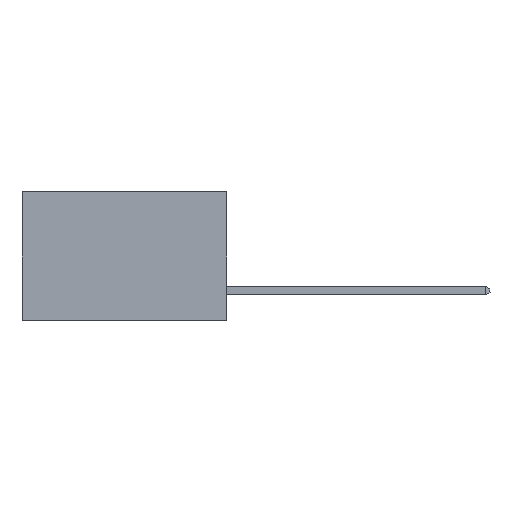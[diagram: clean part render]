
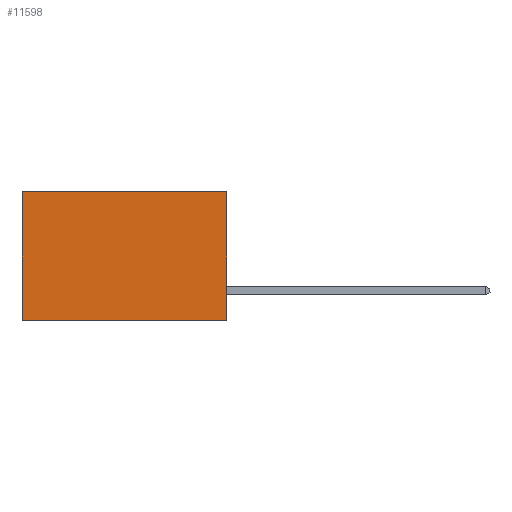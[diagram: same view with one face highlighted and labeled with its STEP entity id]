
A CAD part, left-side view. The second image highlights one B-rep face of the part: STEP entity #11598.
In plain terms, the highlighted planar face has unit normal (-1, 0, 0).
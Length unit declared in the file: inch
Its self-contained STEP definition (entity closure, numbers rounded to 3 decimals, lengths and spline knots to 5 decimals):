
#494 = VERTEX_POINT ( 'NONE', #1465 ) ;
#564 = EDGE_LOOP ( 'NONE', ( #7076, #9869, #7404, #1707 ) ) ;
#666 = EDGE_CURVE ( 'NONE', #3125, #494, #12591, .T. ) ;
#913 = CARTESIAN_POINT ( 'NONE',  ( 0.277, 0., -0.37 ) ) ;
#1465 = CARTESIAN_POINT ( 'NONE',  ( 0.277, 0.59, -0.37 ) ) ;
#1583 = DIRECTION ( 'NONE',  ( 0., 1., 0. ) ) ;
#1707 = ORIENTED_EDGE ( 'NONE', *, *, #13113, .T. ) ;
#2767 = CARTESIAN_POINT ( 'NONE',  ( 0.277, 0., 0. ) ) ;
#3125 = VERTEX_POINT ( 'NONE', #10188 ) ;
#3278 = DIRECTION ( 'NONE',  ( 0., 0., -1. ) ) ;
#3287 = VECTOR ( 'NONE', #5679, 39.37008 ) ;
#3645 = AXIS2_PLACEMENT_3D ( 'NONE', #913, #9851, #3278 ) ;
#3922 = VECTOR ( 'NONE', #1583, 39.37008 ) ;
#4216 = DIRECTION ( 'NONE',  ( 0., 0., -1. ) ) ;
#4463 = DIRECTION ( 'NONE',  ( 0., 1., 0. ) ) ;
#5421 = CARTESIAN_POINT ( 'NONE',  ( 0.277, 0.59, -0.37 ) ) ;
#5566 = PLANE ( 'NONE',  #3645 ) ;
#5643 = EDGE_CURVE ( 'NONE', #9479, #494, #6677, .T. ) ;
#5679 = DIRECTION ( 'NONE',  ( 0., 0., -1. ) ) ;
#5694 = CARTESIAN_POINT ( 'NONE',  ( 0.277, 0., -0.37 ) ) ;
#6456 = VERTEX_POINT ( 'NONE', #9516 ) ;
#6677 = LINE ( 'NONE', #5421, #3287 ) ;
#7076 = ORIENTED_EDGE ( 'NONE', *, *, #5643, .T. ) ;
#7093 = VECTOR ( 'NONE', #4463, 39.37008 ) ;
#7404 = ORIENTED_EDGE ( 'NONE', *, *, #12650, .F. ) ;
#7953 = VECTOR ( 'NONE', #4216, 39.37008 ) ;
#9479 = VERTEX_POINT ( 'NONE', #9644 ) ;
#9516 = CARTESIAN_POINT ( 'NONE',  ( 0.277, 0., 0. ) ) ;
#9644 = CARTESIAN_POINT ( 'NONE',  ( 0.277, 0.59, 0. ) ) ;
#9730 = LINE ( 'NONE', #2767, #3922 ) ;
#9851 = DIRECTION ( 'NONE',  ( 1., 0., 0. ) ) ;
#9869 = ORIENTED_EDGE ( 'NONE', *, *, #666, .F. ) ;
#10188 = CARTESIAN_POINT ( 'NONE',  ( 0.277, 0., -0.37 ) ) ;
#10726 = LINE ( 'NONE', #11707, #7953 ) ;
#11551 = FACE_OUTER_BOUND ( 'NONE', #564, .T. ) ;
#11598 = ADVANCED_FACE ( 'NONE', ( #11551 ), #5566, .F. ) ;
#11707 = CARTESIAN_POINT ( 'NONE',  ( 0.277, 0., -0.37 ) ) ;
#12591 = LINE ( 'NONE', #5694, #7093 ) ;
#12650 = EDGE_CURVE ( 'NONE', #6456, #3125, #10726, .T. ) ;
#13113 = EDGE_CURVE ( 'NONE', #6456, #9479, #9730, .T. ) ;
